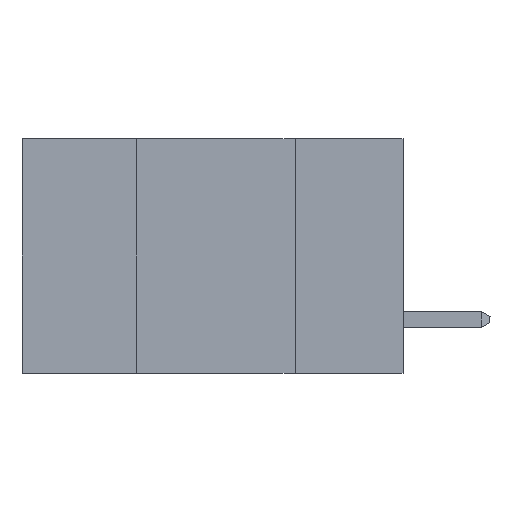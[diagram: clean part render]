
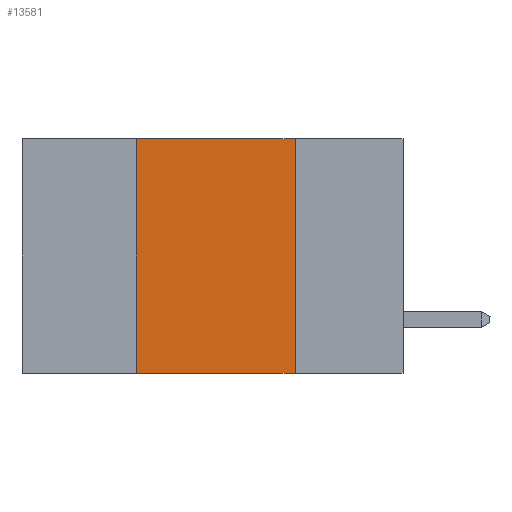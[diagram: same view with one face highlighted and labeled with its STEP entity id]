
A CAD part, left-side view. The second image highlights one B-rep face of the part: STEP entity #13581.
In plain terms, the highlighted planar face has unit normal (-1, 0, 0).
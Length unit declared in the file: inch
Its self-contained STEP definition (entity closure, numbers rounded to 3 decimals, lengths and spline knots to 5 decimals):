
#928 = PLANE ( 'NONE',  #13062 ) ;
#1110 = ORIENTED_EDGE ( 'NONE', *, *, #12783, .T. ) ;
#1559 = CARTESIAN_POINT ( 'NONE',  ( 0., 0.42, 0. ) ) ;
#1705 = VECTOR ( 'NONE', #14047, 39.37008 ) ;
#1835 = LINE ( 'NONE', #13955, #9529 ) ;
#1976 = ORIENTED_EDGE ( 'NONE', *, *, #8587, .F. ) ;
#4206 = CARTESIAN_POINT ( 'NONE',  ( 0., 0.6, 0. ) ) ;
#4285 = DIRECTION ( 'NONE',  ( 0., -1., 0. ) ) ;
#4288 = CARTESIAN_POINT ( 'NONE',  ( 0., 0.6, -0.37 ) ) ;
#4619 = VERTEX_POINT ( 'NONE', #13009 ) ;
#5092 = VERTEX_POINT ( 'NONE', #11036 ) ;
#5246 = CARTESIAN_POINT ( 'NONE',  ( 0., 0.17, 0. ) ) ;
#5826 = EDGE_CURVE ( 'NONE', #4619, #14131, #1835, .T. ) ;
#6707 = EDGE_LOOP ( 'NONE', ( #1976, #7912, #8741, #1110 ) ) ;
#7324 = LINE ( 'NONE', #4206, #7940 ) ;
#7912 = ORIENTED_EDGE ( 'NONE', *, *, #11435, .F. ) ;
#7940 = VECTOR ( 'NONE', #4285, 39.37008 ) ;
#8587 = EDGE_CURVE ( 'NONE', #13326, #5092, #12378, .T. ) ;
#8658 = VECTOR ( 'NONE', #8689, 39.37008 ) ;
#8689 = DIRECTION ( 'NONE',  ( 0., -1., 0. ) ) ;
#8741 = ORIENTED_EDGE ( 'NONE', *, *, #5826, .F. ) ;
#9529 = VECTOR ( 'NONE', #10577, 39.37008 ) ;
#9899 = DIRECTION ( 'NONE',  ( 1., 0., 0. ) ) ;
#10577 = DIRECTION ( 'NONE',  ( 0., 0., 1. ) ) ;
#11036 = CARTESIAN_POINT ( 'NONE',  ( 0., 0.17, -0.37 ) ) ;
#11122 = DIRECTION ( 'NONE',  ( 0., 0., -1. ) ) ;
#11192 = CARTESIAN_POINT ( 'NONE',  ( 0., 0.6, 0. ) ) ;
#11435 = EDGE_CURVE ( 'NONE', #14131, #13326, #7324, .T. ) ;
#12378 = LINE ( 'NONE', #5246, #1705 ) ;
#12783 = EDGE_CURVE ( 'NONE', #4619, #5092, #13028, .T. ) ;
#13009 = CARTESIAN_POINT ( 'NONE',  ( 0., 0.42, -0.37 ) ) ;
#13028 = LINE ( 'NONE', #4288, #8658 ) ;
#13062 = AXIS2_PLACEMENT_3D ( 'NONE', #11192, #9899, #11122 ) ;
#13326 = VERTEX_POINT ( 'NONE', #14232 ) ;
#13581 = ADVANCED_FACE ( 'NONE', ( #13934 ), #928, .F. ) ;
#13934 = FACE_OUTER_BOUND ( 'NONE', #6707, .T. ) ;
#13955 = CARTESIAN_POINT ( 'NONE',  ( 0., 0.42, 0. ) ) ;
#14047 = DIRECTION ( 'NONE',  ( 0., 0., -1. ) ) ;
#14131 = VERTEX_POINT ( 'NONE', #1559 ) ;
#14232 = CARTESIAN_POINT ( 'NONE',  ( 0., 0.17, 0. ) ) ;
